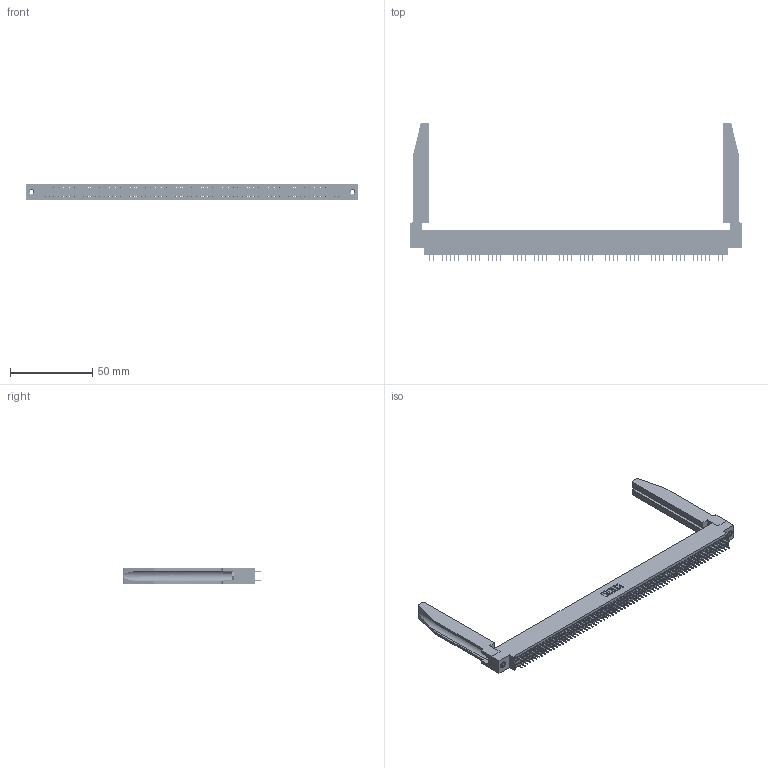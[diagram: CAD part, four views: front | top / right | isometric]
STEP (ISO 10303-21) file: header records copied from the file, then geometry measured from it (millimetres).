
FILE_DESCRIPTION (( 'STEP AP203' ), '1' );
FILE_NAME ('395-142-525-878.STEP', '2020-09-26T07:07:31', ( '' ), ( '' ), 'SwSTEP 2.0', 'SolidWorks 2020', '' );
FILE_SCHEMA (( 'CONFIG_CONTROL_DESIGN' ));
Length unit declared in the file: inch
Products named in the file (5): 345-220-078_345-220-078; 345 Part_0.170 Offset - 0.156 Dia-TH; 345-292-001_345-293-125; 345-250-001_345-250-001-102; 395-142-525-878
Assembly tree (147 placements, depth 2):
  395-142-525-878
    345 Part_0.170 Offset - 0.156 Dia-TH
    345-292-001_345-293-125  x142
    345-250-001_345-250-001-102  x2
    345-220-078_345-220-078  x2
Bounding box: 201.57 x 84 x 9.4 mm (x, y, z)
Volume: 27273.6 mm3; surface area: 35668.3 mm2
Topology: 147 solids, 147 shells, 8032 faces, 22687 edges, 14546 vertices
Faces by surface type: plane 5764, cylinder 2216, bspline 36, cone 12, torus 4
Entity records: 56750 total; most frequent: CARTESIAN_POINT 10403, ORIENTED_EDGE 9234, DIRECTION 8131, EDGE_CURVE 4617, LINE 4111, VECTOR 4111, VERTEX_POINT 3068, AXIS2_PLACEMENT_3D 2010
